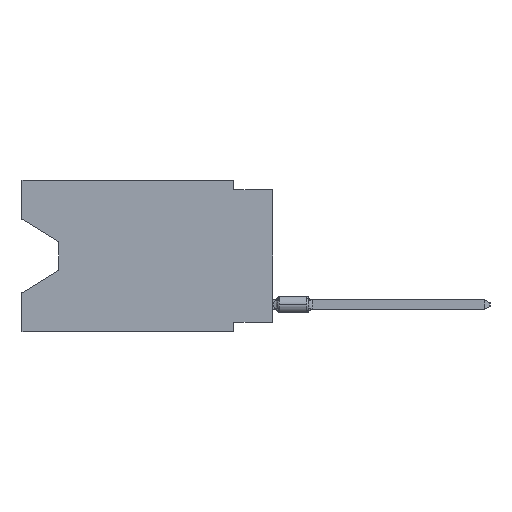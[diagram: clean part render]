
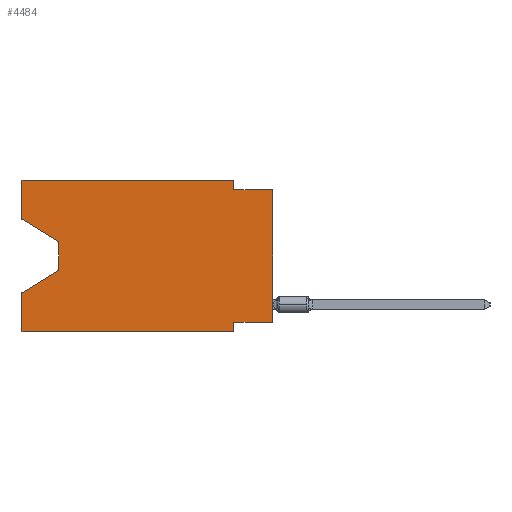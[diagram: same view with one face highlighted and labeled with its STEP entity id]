
A CAD part, left-side view. The second image highlights one B-rep face of the part: STEP entity #4484.
In plain terms, the highlighted planar face has unit normal (-1, 0, 0).
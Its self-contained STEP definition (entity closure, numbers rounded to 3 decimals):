
#294 = VERTEX_POINT ( 'NONE', #19165 ) ;
#297 = VERTEX_POINT ( 'NONE', #14412 ) ;
#841 = EDGE_CURVE ( 'NONE', #2239, #31201, #31141, .T. ) ;
#1431 = VECTOR ( 'NONE', #23982, 1000. ) ;
#2239 = VERTEX_POINT ( 'NONE', #20508 ) ;
#2398 = DIRECTION ( 'NONE',  ( 1., 0., 0. ) ) ;
#2774 = ORIENTED_EDGE ( 'NONE', *, *, #21167, .F. ) ;
#3228 = VERTEX_POINT ( 'NONE', #25043 ) ;
#3322 = DIRECTION ( 'NONE',  ( 0., 0., 1. ) ) ;
#4484 = ADVANCED_FACE ( 'NONE', ( #10464 ), #5151, .F. ) ;
#4713 = DIRECTION ( 'NONE',  ( 0., 0.855, -0.519 ) ) ;
#5109 = CARTESIAN_POINT ( 'NONE',  ( 0., 16.383, -7.36 ) ) ;
#5114 = LINE ( 'NONE', #16620, #30202 ) ;
#5151 = PLANE ( 'NONE',  #13405 ) ;
#5226 = ORIENTED_EDGE ( 'NONE', *, *, #26500, .F. ) ;
#5693 = VERTEX_POINT ( 'NONE', #27368 ) ;
#5787 = LINE ( 'NONE', #25307, #14005 ) ;
#5901 = ORIENTED_EDGE ( 'NONE', *, *, #30306, .T. ) ;
#6105 = DIRECTION ( 'NONE',  ( 0., 0., 1. ) ) ;
#6159 = DIRECTION ( 'NONE',  ( 0., 0., -1. ) ) ;
#6246 = CARTESIAN_POINT ( 'NONE',  ( 0., 16.383, 0. ) ) ;
#6728 = EDGE_CURVE ( 'NONE', #3228, #294, #32733, .T. ) ;
#7354 = LINE ( 'NONE', #30133, #23533 ) ;
#8230 = VERTEX_POINT ( 'NONE', #29552 ) ;
#8669 = LINE ( 'NONE', #11225, #13644 ) ;
#8707 = DIRECTION ( 'NONE',  ( 0., 0., 1. ) ) ;
#8734 = ORIENTED_EDGE ( 'NONE', *, *, #15821, .F. ) ;
#9273 = DIRECTION ( 'NONE',  ( 0., 1., 0. ) ) ;
#9335 = ORIENTED_EDGE ( 'NONE', *, *, #18506, .F. ) ;
#9478 = CARTESIAN_POINT ( 'NONE',  ( 0., 0., -9.271 ) ) ;
#9676 = EDGE_LOOP ( 'NONE', ( #5901, #27614, #30301, #32806, #12859, #30347, #9335, #22808, #8734, #5226, #26507, #2774 ) ) ;
#10270 = DIRECTION ( 'NONE',  ( 0., -1., 0. ) ) ;
#10464 = FACE_OUTER_BOUND ( 'NONE', #9676, .T. ) ;
#11082 = DIRECTION ( 'NONE',  ( 0., -0.855, -0.519 ) ) ;
#11225 = CARTESIAN_POINT ( 'NONE',  ( 0., 16.383, 0. ) ) ;
#12002 = CARTESIAN_POINT ( 'NONE',  ( 0., 0., -9.271 ) ) ;
#12188 = LINE ( 'NONE', #12002, #13021 ) ;
#12859 = ORIENTED_EDGE ( 'NONE', *, *, #21428, .T. ) ;
#13021 = VECTOR ( 'NONE', #9273, 1000. ) ;
#13032 = CARTESIAN_POINT ( 'NONE',  ( 0., 13.97, -4.013 ) ) ;
#13405 = AXIS2_PLACEMENT_3D ( 'NONE', #33059, #2398, #35978 ) ;
#13644 = VECTOR ( 'NONE', #6105, 1000. ) ;
#14005 = VECTOR ( 'NONE', #11082, 1000. ) ;
#14179 = LINE ( 'NONE', #28223, #26612 ) ;
#14412 = CARTESIAN_POINT ( 'NONE',  ( 0., 13.97, -4.013 ) ) ;
#14659 = VERTEX_POINT ( 'NONE', #5109 ) ;
#14897 = CARTESIAN_POINT ( 'NONE',  ( 0., 0., -0.635 ) ) ;
#15291 = CARTESIAN_POINT ( 'NONE',  ( 0., 2.54, -9.906 ) ) ;
#15398 = LINE ( 'NONE', #13032, #1431 ) ;
#15821 = EDGE_CURVE ( 'NONE', #8230, #25273, #5114, .T. ) ;
#16620 = CARTESIAN_POINT ( 'NONE',  ( 0., 0., -0.635 ) ) ;
#17646 = CARTESIAN_POINT ( 'NONE',  ( 0., 2.54, -9.906 ) ) ;
#17812 = LINE ( 'NONE', #26229, #34864 ) ;
#17996 = DIRECTION ( 'NONE',  ( 0., 0., -1. ) ) ;
#18506 = EDGE_CURVE ( 'NONE', #24788, #2239, #12188, .T. ) ;
#18974 = VECTOR ( 'NONE', #3322, 1000. ) ;
#19165 = CARTESIAN_POINT ( 'NONE',  ( 0., 2.54, 0. ) ) ;
#19178 = DIRECTION ( 'NONE',  ( 0., -1., 0. ) ) ;
#19334 = VECTOR ( 'NONE', #21618, 1000. ) ;
#20226 = EDGE_CURVE ( 'NONE', #297, #21688, #15398, .T. ) ;
#20508 = CARTESIAN_POINT ( 'NONE',  ( 0., 2.54, -9.271 ) ) ;
#20948 = EDGE_CURVE ( 'NONE', #21688, #14659, #21138, .T. ) ;
#21138 = LINE ( 'NONE', #24915, #24384 ) ;
#21167 = EDGE_CURVE ( 'NONE', #5693, #3228, #8669, .T. ) ;
#21428 = EDGE_CURVE ( 'NONE', #29713, #31201, #7354, .T. ) ;
#21618 = DIRECTION ( 'NONE',  ( 0., -1., 0. ) ) ;
#21688 = VERTEX_POINT ( 'NONE', #26263 ) ;
#22724 = EDGE_CURVE ( 'NONE', #29713, #14659, #31225, .T. ) ;
#22808 = ORIENTED_EDGE ( 'NONE', *, *, #32624, .T. ) ;
#23533 = VECTOR ( 'NONE', #10270, 1000. ) ;
#23982 = DIRECTION ( 'NONE',  ( 0., 0., -1. ) ) ;
#24384 = VECTOR ( 'NONE', #4713, 1000. ) ;
#24788 = VERTEX_POINT ( 'NONE', #9478 ) ;
#24915 = CARTESIAN_POINT ( 'NONE',  ( 0., 13.97, -5.893 ) ) ;
#25043 = CARTESIAN_POINT ( 'NONE',  ( 0., 16.383, 0. ) ) ;
#25273 = VERTEX_POINT ( 'NONE', #14897 ) ;
#25307 = CARTESIAN_POINT ( 'NONE',  ( 0., 16.383, -2.546 ) ) ;
#26229 = CARTESIAN_POINT ( 'NONE',  ( 0., 2.54, 0. ) ) ;
#26263 = CARTESIAN_POINT ( 'NONE',  ( 0., 13.97, -5.893 ) ) ;
#26500 = EDGE_CURVE ( 'NONE', #294, #8230, #17812, .T. ) ;
#26507 = ORIENTED_EDGE ( 'NONE', *, *, #6728, .F. ) ;
#26612 = VECTOR ( 'NONE', #8707, 1000. ) ;
#27368 = CARTESIAN_POINT ( 'NONE',  ( 0., 16.383, -2.546 ) ) ;
#27614 = ORIENTED_EDGE ( 'NONE', *, *, #20226, .T. ) ;
#28223 = CARTESIAN_POINT ( 'NONE',  ( 0., 0., 0. ) ) ;
#29552 = CARTESIAN_POINT ( 'NONE',  ( 0., 2.54, -0.635 ) ) ;
#29713 = VERTEX_POINT ( 'NONE', #32990 ) ;
#30092 = VECTOR ( 'NONE', #6159, 1000. ) ;
#30133 = CARTESIAN_POINT ( 'NONE',  ( 0., 16.383, -9.906 ) ) ;
#30202 = VECTOR ( 'NONE', #19178, 1000. ) ;
#30301 = ORIENTED_EDGE ( 'NONE', *, *, #20948, .T. ) ;
#30306 = EDGE_CURVE ( 'NONE', #5693, #297, #5787, .T. ) ;
#30347 = ORIENTED_EDGE ( 'NONE', *, *, #841, .F. ) ;
#31141 = LINE ( 'NONE', #17646, #30092 ) ;
#31201 = VERTEX_POINT ( 'NONE', #15291 ) ;
#31225 = LINE ( 'NONE', #6246, #18974 ) ;
#32020 = CARTESIAN_POINT ( 'NONE',  ( 0., 16.383, 0. ) ) ;
#32624 = EDGE_CURVE ( 'NONE', #24788, #25273, #14179, .T. ) ;
#32733 = LINE ( 'NONE', #32020, #19334 ) ;
#32806 = ORIENTED_EDGE ( 'NONE', *, *, #22724, .F. ) ;
#32990 = CARTESIAN_POINT ( 'NONE',  ( 0., 16.383, -9.906 ) ) ;
#33059 = CARTESIAN_POINT ( 'NONE',  ( 0., 16.383, 0. ) ) ;
#34864 = VECTOR ( 'NONE', #17996, 1000. ) ;
#35978 = DIRECTION ( 'NONE',  ( 0., 0., -1. ) ) ;
